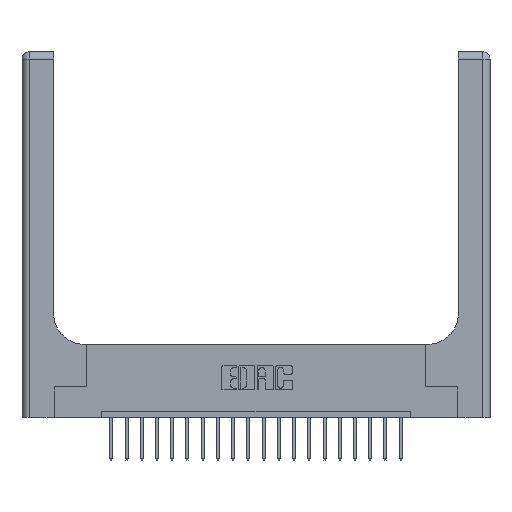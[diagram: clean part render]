
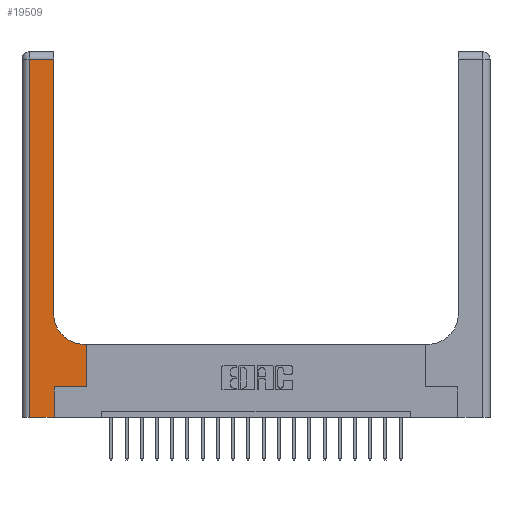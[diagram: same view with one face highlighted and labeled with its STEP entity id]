
A CAD part, top view. The second image highlights one B-rep face of the part: STEP entity #19509.
In plain terms, the highlighted planar face has unit normal (0, 0, 1).
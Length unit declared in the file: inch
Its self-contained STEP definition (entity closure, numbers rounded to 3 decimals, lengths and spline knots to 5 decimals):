
#756 = CARTESIAN_POINT ( 'NONE',  ( 0.51, 0.6, 0.37 ) ) ;
#1715 = AXIS2_PLACEMENT_3D ( 'NONE', #8839, #10655, #8740 ) ;
#2786 = VERTEX_POINT ( 'NONE', #16032 ) ;
#3141 = CARTESIAN_POINT ( 'NONE',  ( 0.528, 0.25, 0.37 ) ) ;
#3232 = EDGE_CURVE ( 'NONE', #7857, #12200, #3296, .T. ) ;
#3296 = LINE ( 'NONE', #19571, #11985 ) ;
#3465 = ORIENTED_EDGE ( 'NONE', *, *, #5298, .T. ) ;
#3824 = CARTESIAN_POINT ( 'NONE',  ( 0.26, 2.94, 0.37 ) ) ;
#3843 = PLANE ( 'NONE',  #1715 ) ;
#3937 = CARTESIAN_POINT ( 'NONE',  ( 0.51, 0.85, 0.37 ) ) ;
#3983 = EDGE_CURVE ( 'NONE', #11366, #7857, #12233, .T. ) ;
#4205 = VERTEX_POINT ( 'NONE', #10017 ) ;
#4253 = CARTESIAN_POINT ( 'NONE',  ( 0.265, 0.25, 0.37 ) ) ;
#4287 = EDGE_CURVE ( 'NONE', #4205, #7789, #11642, .T. ) ;
#4744 = VECTOR ( 'NONE', #14024, 39.37008 ) ;
#4997 = DIRECTION ( 'NONE',  ( 0., 1., 0. ) ) ;
#5298 = EDGE_CURVE ( 'NONE', #17313, #11366, #7052, .T. ) ;
#5507 = CARTESIAN_POINT ( 'NONE',  ( 0.06, 0., 0.37 ) ) ;
#5511 = CARTESIAN_POINT ( 'NONE',  ( 0.06, 2.94, 0.37 ) ) ;
#5937 = DIRECTION ( 'NONE',  ( 0., 1., 0. ) ) ;
#6076 = LINE ( 'NONE', #4253, #4744 ) ;
#6220 = ORIENTED_EDGE ( 'NONE', *, *, #3983, .T. ) ;
#7033 = CARTESIAN_POINT ( 'NONE',  ( 0.528, 0.25, 0.37 ) ) ;
#7042 = VERTEX_POINT ( 'NONE', #7033 ) ;
#7052 = LINE ( 'NONE', #7370, #9659 ) ;
#7150 = DIRECTION ( 'NONE',  ( 1., 0., 0. ) ) ;
#7370 = CARTESIAN_POINT ( 'NONE',  ( 0.06, 3., 0.37 ) ) ;
#7542 = ORIENTED_EDGE ( 'NONE', *, *, #18599, .T. ) ;
#7561 = ORIENTED_EDGE ( 'NONE', *, *, #12102, .T. ) ;
#7789 = VERTEX_POINT ( 'NONE', #756 ) ;
#7857 = VERTEX_POINT ( 'NONE', #14113 ) ;
#7881 = VECTOR ( 'NONE', #5937, 39.37008 ) ;
#8653 = ORIENTED_EDGE ( 'NONE', *, *, #4287, .T. ) ;
#8740 = DIRECTION ( 'NONE',  ( -1., 0., 0. ) ) ;
#8839 = CARTESIAN_POINT ( 'NONE',  ( 0., 3., 0.37 ) ) ;
#9399 = VECTOR ( 'NONE', #11233, 39.37008 ) ;
#9659 = VECTOR ( 'NONE', #13820, 39.37008 ) ;
#9868 = CARTESIAN_POINT ( 'NONE',  ( 0.265, 0.25, 0.37 ) ) ;
#10017 = CARTESIAN_POINT ( 'NONE',  ( 0.528, 0.6, 0.37 ) ) ;
#10190 = LINE ( 'NONE', #11331, #14292 ) ;
#10655 = DIRECTION ( 'NONE',  ( 0., 0., -1. ) ) ;
#10929 = VERTEX_POINT ( 'NONE', #3824 ) ;
#11209 = ORIENTED_EDGE ( 'NONE', *, *, #11225, .T. ) ;
#11225 = EDGE_CURVE ( 'NONE', #7789, #2786, #13875, .T. ) ;
#11233 = DIRECTION ( 'NONE',  ( 0., 1., 0. ) ) ;
#11331 = CARTESIAN_POINT ( 'NONE',  ( 0., 2.94, 0.37 ) ) ;
#11366 = VERTEX_POINT ( 'NONE', #5507 ) ;
#11642 = LINE ( 'NONE', #11962, #14244 ) ;
#11962 = CARTESIAN_POINT ( 'NONE',  ( 0.26, 0.6, 0.37 ) ) ;
#11985 = VECTOR ( 'NONE', #4997, 39.37008 ) ;
#12102 = EDGE_CURVE ( 'NONE', #10929, #17313, #10190, .T. ) ;
#12200 = VERTEX_POINT ( 'NONE', #9868 ) ;
#12233 = LINE ( 'NONE', #13922, #14225 ) ;
#13463 = EDGE_CURVE ( 'NONE', #12200, #7042, #6076, .T. ) ;
#13820 = DIRECTION ( 'NONE',  ( 0., -1., 0. ) ) ;
#13875 = CIRCLE ( 'NONE', #16601, 0.25 ) ;
#13904 = DIRECTION ( 'NONE',  ( 0., 0., -1. ) ) ;
#13922 = CARTESIAN_POINT ( 'NONE',  ( 0., 0., 0.37 ) ) ;
#14024 = DIRECTION ( 'NONE',  ( 1., 0., 0. ) ) ;
#14113 = CARTESIAN_POINT ( 'NONE',  ( 0.265, 0., 0.37 ) ) ;
#14225 = VECTOR ( 'NONE', #7150, 39.37008 ) ;
#14244 = VECTOR ( 'NONE', #18150, 39.37008 ) ;
#14292 = VECTOR ( 'NONE', #14739, 39.37008 ) ;
#14443 = CARTESIAN_POINT ( 'NONE',  ( 0.26, 3., 0.37 ) ) ;
#14579 = EDGE_LOOP ( 'NONE', ( #7542, #7561, #3465, #6220, #18782, #20254, #20948, #8653, #11209 ) ) ;
#14739 = DIRECTION ( 'NONE',  ( -1., 0., 0. ) ) ;
#14759 = LINE ( 'NONE', #14443, #9399 ) ;
#16032 = CARTESIAN_POINT ( 'NONE',  ( 0.26, 0.85, 0.37 ) ) ;
#16601 = AXIS2_PLACEMENT_3D ( 'NONE', #3937, #13904, #17212 ) ;
#17026 = FACE_OUTER_BOUND ( 'NONE', #14579, .T. ) ;
#17212 = DIRECTION ( 'NONE',  ( 1., 0., 0. ) ) ;
#17313 = VERTEX_POINT ( 'NONE', #5511 ) ;
#18150 = DIRECTION ( 'NONE',  ( -1., 0., 0. ) ) ;
#18599 = EDGE_CURVE ( 'NONE', #2786, #10929, #14759, .T. ) ;
#18782 = ORIENTED_EDGE ( 'NONE', *, *, #3232, .T. ) ;
#19509 = ADVANCED_FACE ( 'NONE', ( #17026 ), #3843, .F. ) ;
#19571 = CARTESIAN_POINT ( 'NONE',  ( 0.265, 0., 0.37 ) ) ;
#20254 = ORIENTED_EDGE ( 'NONE', *, *, #13463, .T. ) ;
#20707 = EDGE_CURVE ( 'NONE', #7042, #4205, #20921, .T. ) ;
#20921 = LINE ( 'NONE', #3141, #7881 ) ;
#20948 = ORIENTED_EDGE ( 'NONE', *, *, #20707, .T. ) ;
